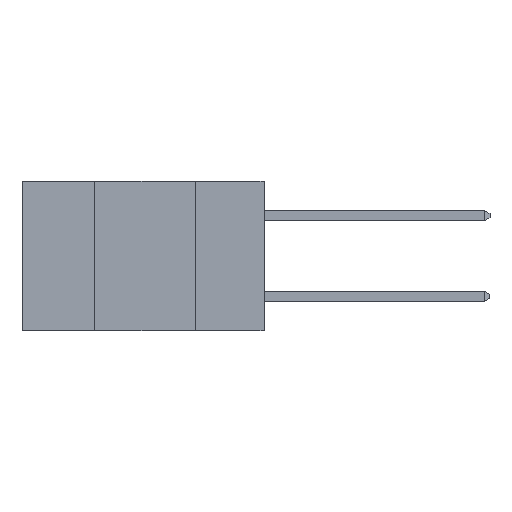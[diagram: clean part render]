
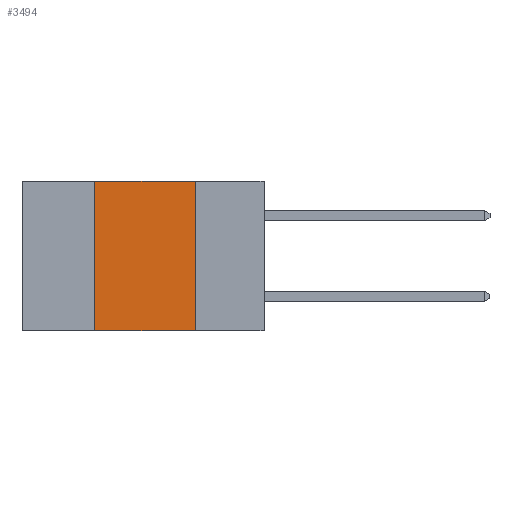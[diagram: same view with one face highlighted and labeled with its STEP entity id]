
A CAD part, left-side view. The second image highlights one B-rep face of the part: STEP entity #3494.
In plain terms, the highlighted planar face has unit normal (-1, 0, 0).
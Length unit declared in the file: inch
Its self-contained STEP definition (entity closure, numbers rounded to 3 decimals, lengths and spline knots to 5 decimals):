
#672 = DIRECTION ( 'NONE',  ( 0., 0., -1. ) ) ;
#3046 = CARTESIAN_POINT ( 'NONE',  ( 0., 0.17, 0. ) ) ;
#3088 = VERTEX_POINT ( 'NONE', #12259 ) ;
#3494 = ADVANCED_FACE ( 'NONE', ( #23429 ), #22178, .F. ) ;
#3605 = DIRECTION ( 'NONE',  ( 0., 0., -1. ) ) ;
#3804 = CARTESIAN_POINT ( 'NONE',  ( 0., 0.6, 0. ) ) ;
#4023 = VERTEX_POINT ( 'NONE', #29045 ) ;
#4674 = ORIENTED_EDGE ( 'NONE', *, *, #13679, .T. ) ;
#6065 = CARTESIAN_POINT ( 'NONE',  ( 0., 0.17, -0.37 ) ) ;
#7063 = LINE ( 'NONE', #3046, #16506 ) ;
#8177 = EDGE_LOOP ( 'NONE', ( #29582, #10867, #9396, #4674 ) ) ;
#8420 = EDGE_CURVE ( 'NONE', #4023, #9344, #15814, .T. ) ;
#8986 = DIRECTION ( 'NONE',  ( 0., 0., 1. ) ) ;
#9344 = VERTEX_POINT ( 'NONE', #14527 ) ;
#9396 = ORIENTED_EDGE ( 'NONE', *, *, #8420, .F. ) ;
#10867 = ORIENTED_EDGE ( 'NONE', *, *, #29576, .F. ) ;
#12259 = CARTESIAN_POINT ( 'NONE',  ( 0., 0.17, 0. ) ) ;
#12552 = VECTOR ( 'NONE', #29160, 39.37008 ) ;
#13156 = VECTOR ( 'NONE', #20083, 39.37008 ) ;
#13679 = EDGE_CURVE ( 'NONE', #4023, #21780, #24834, .T. ) ;
#14527 = CARTESIAN_POINT ( 'NONE',  ( 0., 0.42, 0. ) ) ;
#15417 = CARTESIAN_POINT ( 'NONE',  ( 0., 0.6, 0. ) ) ;
#15814 = LINE ( 'NONE', #25186, #21228 ) ;
#16506 = VECTOR ( 'NONE', #672, 39.37008 ) ;
#16541 = AXIS2_PLACEMENT_3D ( 'NONE', #15417, #24516, #3605 ) ;
#20083 = DIRECTION ( 'NONE',  ( 0., -1., 0. ) ) ;
#21228 = VECTOR ( 'NONE', #8986, 39.37008 ) ;
#21780 = VERTEX_POINT ( 'NONE', #6065 ) ;
#22178 = PLANE ( 'NONE',  #16541 ) ;
#22968 = EDGE_CURVE ( 'NONE', #3088, #21780, #7063, .T. ) ;
#23429 = FACE_OUTER_BOUND ( 'NONE', #8177, .T. ) ;
#24000 = LINE ( 'NONE', #3804, #13156 ) ;
#24516 = DIRECTION ( 'NONE',  ( 1., 0., 0. ) ) ;
#24574 = CARTESIAN_POINT ( 'NONE',  ( 0., 0.6, -0.37 ) ) ;
#24834 = LINE ( 'NONE', #24574, #12552 ) ;
#25186 = CARTESIAN_POINT ( 'NONE',  ( 0., 0.42, 0. ) ) ;
#29045 = CARTESIAN_POINT ( 'NONE',  ( 0., 0.42, -0.37 ) ) ;
#29160 = DIRECTION ( 'NONE',  ( 0., -1., 0. ) ) ;
#29576 = EDGE_CURVE ( 'NONE', #9344, #3088, #24000, .T. ) ;
#29582 = ORIENTED_EDGE ( 'NONE', *, *, #22968, .F. ) ;
